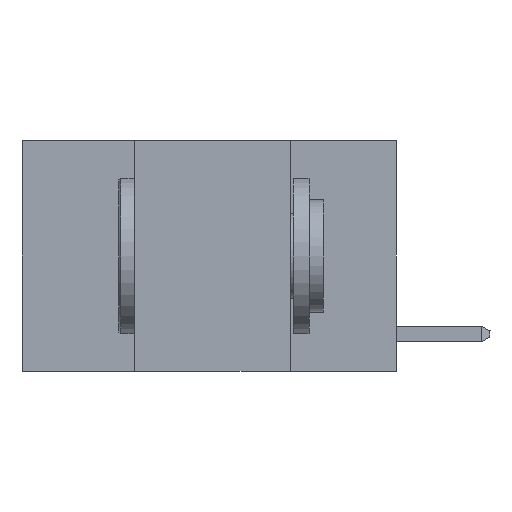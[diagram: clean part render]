
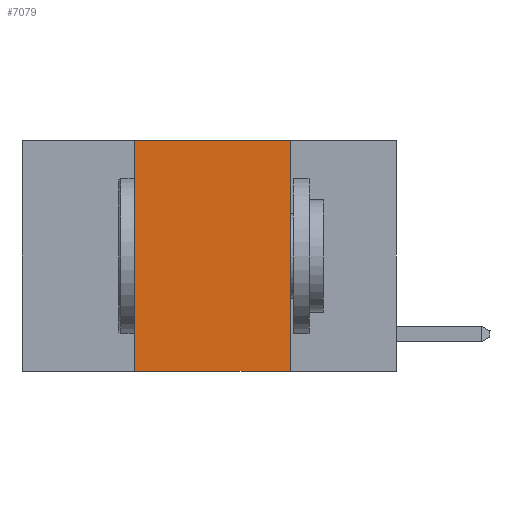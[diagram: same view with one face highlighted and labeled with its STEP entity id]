
A CAD part, left-side view. The second image highlights one B-rep face of the part: STEP entity #7079.
In plain terms, the highlighted planar face has unit normal (-1, 0, 0).
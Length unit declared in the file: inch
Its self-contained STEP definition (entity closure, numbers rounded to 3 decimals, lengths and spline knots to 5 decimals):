
#5035 = EDGE_LOOP ( 'NONE', ( #24957, #22643, #5520, #11732 ) ) ;
#5520 = ORIENTED_EDGE ( 'NONE', *, *, #6838, .F. ) ;
#6830 = LINE ( 'NONE', #22160, #22025 ) ;
#6838 = EDGE_CURVE ( 'NONE', #16034, #17129, #28030, .T. ) ;
#7079 = ADVANCED_FACE ( 'NONE', ( #24807 ), #8475, .F. ) ;
#7227 = CARTESIAN_POINT ( 'NONE',  ( 0., 0.42, 0. ) ) ;
#7313 = CARTESIAN_POINT ( 'NONE',  ( 0., 0.17, 0. ) ) ;
#7386 = CARTESIAN_POINT ( 'NONE',  ( 0., 0.6, 0. ) ) ;
#7872 = CARTESIAN_POINT ( 'NONE',  ( 0., 0.17, -0.37 ) ) ;
#8475 = PLANE ( 'NONE',  #15488 ) ;
#9962 = CARTESIAN_POINT ( 'NONE',  ( 0., 0.17, 0. ) ) ;
#11732 = ORIENTED_EDGE ( 'NONE', *, *, #18299, .T. ) ;
#11768 = VECTOR ( 'NONE', #11964, 39.37008 ) ;
#11964 = DIRECTION ( 'NONE',  ( 0., 0., 1. ) ) ;
#15488 = AXIS2_PLACEMENT_3D ( 'NONE', #23984, #17404, #24090 ) ;
#16034 = VERTEX_POINT ( 'NONE', #28713 ) ;
#16396 = EDGE_CURVE ( 'NONE', #19297, #22130, #21825, .T. ) ;
#16893 = VECTOR ( 'NONE', #23228, 39.37008 ) ;
#17129 = VERTEX_POINT ( 'NONE', #26071 ) ;
#17404 = DIRECTION ( 'NONE',  ( 1., 0., 0. ) ) ;
#18299 = EDGE_CURVE ( 'NONE', #16034, #22130, #6830, .T. ) ;
#19297 = VERTEX_POINT ( 'NONE', #9962 ) ;
#20117 = EDGE_CURVE ( 'NONE', #17129, #19297, #22321, .T. ) ;
#21825 = LINE ( 'NONE', #7313, #16893 ) ;
#22025 = VECTOR ( 'NONE', #26310, 39.37008 ) ;
#22130 = VERTEX_POINT ( 'NONE', #7872 ) ;
#22160 = CARTESIAN_POINT ( 'NONE',  ( 0., 0.6, -0.37 ) ) ;
#22321 = LINE ( 'NONE', #7386, #28012 ) ;
#22643 = ORIENTED_EDGE ( 'NONE', *, *, #20117, .F. ) ;
#23228 = DIRECTION ( 'NONE',  ( 0., 0., -1. ) ) ;
#23984 = CARTESIAN_POINT ( 'NONE',  ( 0., 0.6, 0. ) ) ;
#24090 = DIRECTION ( 'NONE',  ( 0., 0., -1. ) ) ;
#24807 = FACE_OUTER_BOUND ( 'NONE', #5035, .T. ) ;
#24957 = ORIENTED_EDGE ( 'NONE', *, *, #16396, .F. ) ;
#26071 = CARTESIAN_POINT ( 'NONE',  ( 0., 0.42, 0. ) ) ;
#26310 = DIRECTION ( 'NONE',  ( 0., -1., 0. ) ) ;
#27956 = DIRECTION ( 'NONE',  ( 0., -1., 0. ) ) ;
#28012 = VECTOR ( 'NONE', #27956, 39.37008 ) ;
#28030 = LINE ( 'NONE', #7227, #11768 ) ;
#28713 = CARTESIAN_POINT ( 'NONE',  ( 0., 0.42, -0.37 ) ) ;
